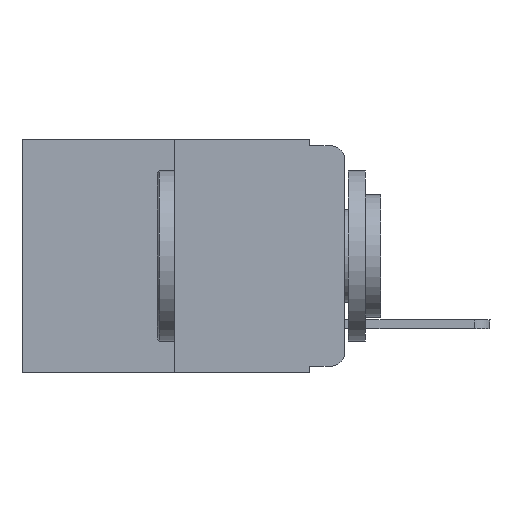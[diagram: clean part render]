
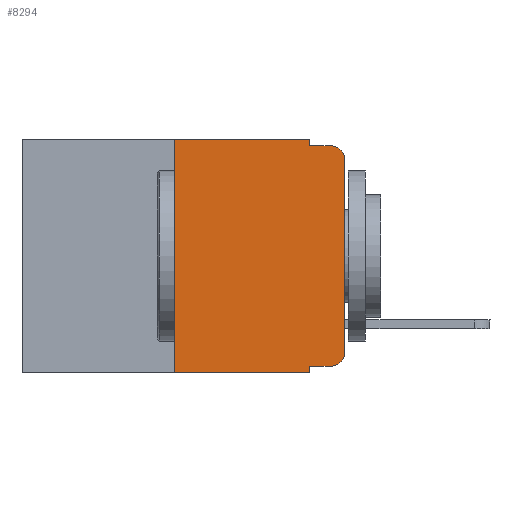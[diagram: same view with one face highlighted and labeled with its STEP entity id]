
A CAD part, left-side view. The second image highlights one B-rep face of the part: STEP entity #8294.
In plain terms, the highlighted planar face has unit normal (-1, 0, 0).
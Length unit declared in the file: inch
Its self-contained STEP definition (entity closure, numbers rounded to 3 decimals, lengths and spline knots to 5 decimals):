
#1 = ORIENTED_EDGE ( 'NONE', *, *, #7867, .T. ) ;
#32 = CARTESIAN_POINT ( 'NONE',  ( 0., 0.051, -0.333 ) ) ;
#123 = CARTESIAN_POINT ( 'NONE',  ( 0., 0.473, 0. ) ) ;
#376 = LINE ( 'NONE', #3663, #7339 ) ;
#405 = CARTESIAN_POINT ( 'NONE',  ( 0., 0.25, 0. ) ) ;
#838 = VECTOR ( 'NONE', #1886, 39.37008 ) ;
#859 = LINE ( 'NONE', #32, #8853 ) ;
#994 = DIRECTION ( 'NONE',  ( 0., 0., -1. ) ) ;
#1004 = EDGE_LOOP ( 'NONE', ( #5431, #5247, #1135, #8987, #10030, #9962, #9330, #5151, #1, #6952 ) ) ;
#1135 = ORIENTED_EDGE ( 'NONE', *, *, #9101, .F. ) ;
#1288 = EDGE_CURVE ( 'NONE', #5586, #7158, #3599, .T. ) ;
#1380 = EDGE_CURVE ( 'NONE', #3189, #8775, #7082, .T. ) ;
#1442 = DIRECTION ( 'NONE',  ( -1., 0., 0. ) ) ;
#1539 = VERTEX_POINT ( 'NONE', #9114 ) ;
#1886 = DIRECTION ( 'NONE',  ( 0., 0., -1. ) ) ;
#1975 = LINE ( 'NONE', #405, #8159 ) ;
#2193 = LINE ( 'NONE', #5472, #6490 ) ;
#2288 = CARTESIAN_POINT ( 'NONE',  ( 0., 0.02, -0.333 ) ) ;
#2500 = VERTEX_POINT ( 'NONE', #7412 ) ;
#2526 = EDGE_CURVE ( 'NONE', #7158, #2500, #9288, .T. ) ;
#2593 = LINE ( 'NONE', #8336, #10015 ) ;
#2706 = PLANE ( 'NONE',  #5954 ) ;
#2889 = VERTEX_POINT ( 'NONE', #7506 ) ;
#3035 = CARTESIAN_POINT ( 'NONE',  ( 0., 0.25, -0.343 ) ) ;
#3094 = CARTESIAN_POINT ( 'NONE',  ( 0., 0.25, 0. ) ) ;
#3171 = DIRECTION ( 'NONE',  ( 0., -1., 0. ) ) ;
#3189 = VERTEX_POINT ( 'NONE', #10299 ) ;
#3212 = CIRCLE ( 'NONE', #5608, 0.02 ) ;
#3426 = DIRECTION ( 'NONE',  ( 1., 0., 0. ) ) ;
#3431 = CARTESIAN_POINT ( 'NONE',  ( 0., 0.051, 0. ) ) ;
#3546 = DIRECTION ( 'NONE',  ( 0., 0., -1. ) ) ;
#3599 = LINE ( 'NONE', #5205, #9901 ) ;
#3663 = CARTESIAN_POINT ( 'NONE',  ( 0., 0.473, -0.343 ) ) ;
#3767 = CARTESIAN_POINT ( 'NONE',  ( 0., 0.051, 0. ) ) ;
#3892 = CARTESIAN_POINT ( 'NONE',  ( 0., 0.02, -0.01 ) ) ;
#4394 = DIRECTION ( 'NONE',  ( -1., 0., 0. ) ) ;
#4604 = DIRECTION ( 'NONE',  ( 0., -1., 0. ) ) ;
#4779 = CARTESIAN_POINT ( 'NONE',  ( 0., 0.02, -0.313 ) ) ;
#5151 = ORIENTED_EDGE ( 'NONE', *, *, #1380, .F. ) ;
#5205 = CARTESIAN_POINT ( 'NONE',  ( 0., 0.473, 0. ) ) ;
#5247 = ORIENTED_EDGE ( 'NONE', *, *, #7601, .T. ) ;
#5248 = DIRECTION ( 'NONE',  ( 0., 0., 1. ) ) ;
#5431 = ORIENTED_EDGE ( 'NONE', *, *, #5912, .T. ) ;
#5472 = CARTESIAN_POINT ( 'NONE',  ( 0., 0.051, -0.01 ) ) ;
#5586 = VERTEX_POINT ( 'NONE', #3094 ) ;
#5608 = AXIS2_PLACEMENT_3D ( 'NONE', #5963, #4394, #3546 ) ;
#5912 = EDGE_CURVE ( 'NONE', #2889, #1539, #2593, .T. ) ;
#5954 = AXIS2_PLACEMENT_3D ( 'NONE', #123, #3426, #994 ) ;
#5957 = DIRECTION ( 'NONE',  ( 0., -1., 0. ) ) ;
#5963 = CARTESIAN_POINT ( 'NONE',  ( 0., 0.02, -0.03 ) ) ;
#6187 = DIRECTION ( 'NONE',  ( 0., 0., 1. ) ) ;
#6490 = VECTOR ( 'NONE', #4604, 39.37008 ) ;
#6853 = EDGE_CURVE ( 'NONE', #8396, #5586, #1975, .T. ) ;
#6935 = DIRECTION ( 'NONE',  ( 0., -1., 0. ) ) ;
#6952 = ORIENTED_EDGE ( 'NONE', *, *, #7841, .T. ) ;
#7082 = LINE ( 'NONE', #9606, #10076 ) ;
#7158 = VERTEX_POINT ( 'NONE', #3431 ) ;
#7245 = DIRECTION ( 'NONE',  ( 0., 0., -1. ) ) ;
#7339 = VECTOR ( 'NONE', #6935, 39.37008 ) ;
#7412 = CARTESIAN_POINT ( 'NONE',  ( 0., 0.051, -0.01 ) ) ;
#7506 = CARTESIAN_POINT ( 'NONE',  ( 0., 0., -0.313 ) ) ;
#7601 = EDGE_CURVE ( 'NONE', #1539, #8344, #3212, .T. ) ;
#7841 = EDGE_CURVE ( 'NONE', #8394, #2889, #8684, .T. ) ;
#7867 = EDGE_CURVE ( 'NONE', #3189, #8394, #859, .T. ) ;
#8159 = VECTOR ( 'NONE', #5248, 39.37008 ) ;
#8294 = ADVANCED_FACE ( 'NONE', ( #10017 ), #2706, .F. ) ;
#8336 = CARTESIAN_POINT ( 'NONE',  ( 0., 0., 0. ) ) ;
#8344 = VERTEX_POINT ( 'NONE', #3892 ) ;
#8394 = VERTEX_POINT ( 'NONE', #2288 ) ;
#8396 = VERTEX_POINT ( 'NONE', #3035 ) ;
#8684 = CIRCLE ( 'NONE', #10408, 0.02 ) ;
#8751 = EDGE_CURVE ( 'NONE', #8396, #8775, #376, .T. ) ;
#8775 = VERTEX_POINT ( 'NONE', #9512 ) ;
#8853 = VECTOR ( 'NONE', #3171, 39.37008 ) ;
#8987 = ORIENTED_EDGE ( 'NONE', *, *, #2526, .F. ) ;
#9101 = EDGE_CURVE ( 'NONE', #2500, #8344, #2193, .T. ) ;
#9114 = CARTESIAN_POINT ( 'NONE',  ( 0., 0., -0.03 ) ) ;
#9288 = LINE ( 'NONE', #3767, #838 ) ;
#9330 = ORIENTED_EDGE ( 'NONE', *, *, #8751, .T. ) ;
#9512 = CARTESIAN_POINT ( 'NONE',  ( 0., 0.051, -0.343 ) ) ;
#9606 = CARTESIAN_POINT ( 'NONE',  ( 0., 0.051, 0. ) ) ;
#9712 = DIRECTION ( 'NONE',  ( 0., 0., -1. ) ) ;
#9901 = VECTOR ( 'NONE', #5957, 39.37008 ) ;
#9962 = ORIENTED_EDGE ( 'NONE', *, *, #6853, .F. ) ;
#10015 = VECTOR ( 'NONE', #6187, 39.37008 ) ;
#10017 = FACE_OUTER_BOUND ( 'NONE', #1004, .T. ) ;
#10030 = ORIENTED_EDGE ( 'NONE', *, *, #1288, .F. ) ;
#10076 = VECTOR ( 'NONE', #9712, 39.37008 ) ;
#10299 = CARTESIAN_POINT ( 'NONE',  ( 0., 0.051, -0.333 ) ) ;
#10408 = AXIS2_PLACEMENT_3D ( 'NONE', #4779, #1442, #7245 ) ;
